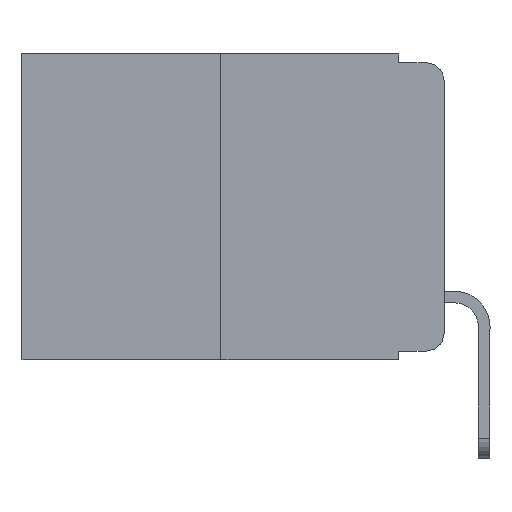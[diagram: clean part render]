
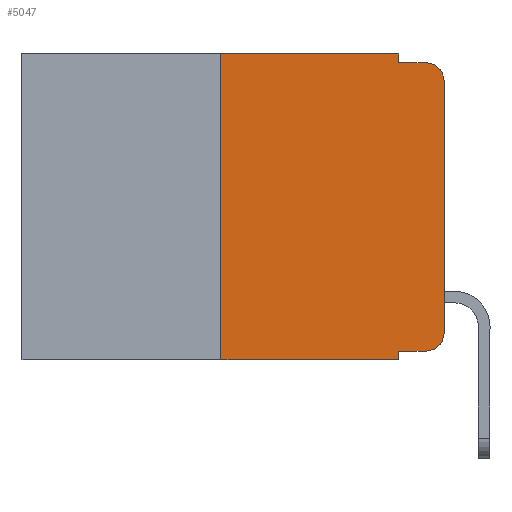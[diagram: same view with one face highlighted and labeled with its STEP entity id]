
A CAD part, left-side view. The second image highlights one B-rep face of the part: STEP entity #5047.
In plain terms, the highlighted planar face has unit normal (-1, 0, 0).
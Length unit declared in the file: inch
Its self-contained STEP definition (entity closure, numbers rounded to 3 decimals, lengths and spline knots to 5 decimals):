
#121 = VERTEX_POINT ( 'NONE', #5667 ) ;
#524 = LINE ( 'NONE', #859, #8742 ) ;
#543 = DIRECTION ( 'NONE',  ( -1., 0., 0. ) ) ;
#813 = DIRECTION ( 'NONE',  ( 0., 0., -1. ) ) ;
#859 = CARTESIAN_POINT ( 'NONE',  ( 0., 0.473, 0. ) ) ;
#891 = DIRECTION ( 'NONE',  ( 0., 0., -1. ) ) ;
#1900 = VERTEX_POINT ( 'NONE', #12485 ) ;
#2143 = LINE ( 'NONE', #16636, #10209 ) ;
#2450 = CARTESIAN_POINT ( 'NONE',  ( 0., 0.051, -0.01 ) ) ;
#2594 = ORIENTED_EDGE ( 'NONE', *, *, #8922, .F. ) ;
#2595 = DIRECTION ( 'NONE',  ( 1., 0., 0. ) ) ;
#3154 = VERTEX_POINT ( 'NONE', #13606 ) ;
#3578 = VERTEX_POINT ( 'NONE', #2450 ) ;
#3741 = LINE ( 'NONE', #18956, #18995 ) ;
#3841 = CARTESIAN_POINT ( 'NONE',  ( 0., 0.02, -0.01 ) ) ;
#3897 = AXIS2_PLACEMENT_3D ( 'NONE', #10343, #543, #11857 ) ;
#4141 = CARTESIAN_POINT ( 'NONE',  ( 0., 0.02, -0.03 ) ) ;
#4151 = ORIENTED_EDGE ( 'NONE', *, *, #8926, .F. ) ;
#5047 = ADVANCED_FACE ( 'NONE', ( #7954 ), #5959, .F. ) ;
#5652 = CARTESIAN_POINT ( 'NONE',  ( 0., 0.25, -0.343 ) ) ;
#5667 = CARTESIAN_POINT ( 'NONE',  ( 0., 0., -0.313 ) ) ;
#5697 = CARTESIAN_POINT ( 'NONE',  ( 0., 0., 0. ) ) ;
#5762 = DIRECTION ( 'NONE',  ( 0., 0., -1. ) ) ;
#5907 = CARTESIAN_POINT ( 'NONE',  ( 0., 0.051, -0.333 ) ) ;
#5959 = PLANE ( 'NONE',  #12268 ) ;
#6906 = ORIENTED_EDGE ( 'NONE', *, *, #8038, .F. ) ;
#7198 = VECTOR ( 'NONE', #7282, 39.37008 ) ;
#7282 = DIRECTION ( 'NONE',  ( 0., 0., 1. ) ) ;
#7420 = CARTESIAN_POINT ( 'NONE',  ( 0., 0.25, 0. ) ) ;
#7494 = VERTEX_POINT ( 'NONE', #10659 ) ;
#7954 = FACE_OUTER_BOUND ( 'NONE', #16239, .T. ) ;
#8038 = EDGE_CURVE ( 'NONE', #1900, #3154, #524, .T. ) ;
#8399 = ORIENTED_EDGE ( 'NONE', *, *, #8951, .T. ) ;
#8606 = LINE ( 'NONE', #7420, #13829 ) ;
#8622 = EDGE_CURVE ( 'NONE', #10189, #7494, #2143, .T. ) ;
#8742 = VECTOR ( 'NONE', #18988, 39.37008 ) ;
#8869 = EDGE_CURVE ( 'NONE', #121, #16444, #15114, .T. ) ;
#8894 = EDGE_CURVE ( 'NONE', #16444, #18422, #14265, .T. ) ;
#8897 = EDGE_CURVE ( 'NONE', #3578, #18422, #17869, .T. ) ;
#8922 = EDGE_CURVE ( 'NONE', #3154, #3578, #9420, .T. ) ;
#8925 = EDGE_CURVE ( 'NONE', #10189, #1900, #8606, .T. ) ;
#8926 = EDGE_CURVE ( 'NONE', #9802, #7494, #3741, .T. ) ;
#8951 = EDGE_CURVE ( 'NONE', #9802, #10324, #11674, .T. ) ;
#8952 = EDGE_CURVE ( 'NONE', #10324, #121, #14954, .T. ) ;
#9005 = DIRECTION ( 'NONE',  ( 0., 0., 1. ) ) ;
#9420 = LINE ( 'NONE', #13471, #17021 ) ;
#9636 = ORIENTED_EDGE ( 'NONE', *, *, #8869, .T. ) ;
#9802 = VERTEX_POINT ( 'NONE', #10296 ) ;
#10137 = ORIENTED_EDGE ( 'NONE', *, *, #8894, .T. ) ;
#10189 = VERTEX_POINT ( 'NONE', #5652 ) ;
#10209 = VECTOR ( 'NONE', #18006, 39.37008 ) ;
#10296 = CARTESIAN_POINT ( 'NONE',  ( 0., 0.051, -0.333 ) ) ;
#10324 = VERTEX_POINT ( 'NONE', #10920 ) ;
#10343 = CARTESIAN_POINT ( 'NONE',  ( 0., 0.02, -0.313 ) ) ;
#10659 = CARTESIAN_POINT ( 'NONE',  ( 0., 0.051, -0.343 ) ) ;
#10920 = CARTESIAN_POINT ( 'NONE',  ( 0., 0.02, -0.333 ) ) ;
#11218 = VECTOR ( 'NONE', #13531, 39.37008 ) ;
#11576 = ORIENTED_EDGE ( 'NONE', *, *, #8925, .F. ) ;
#11674 = LINE ( 'NONE', #5907, #11218 ) ;
#11857 = DIRECTION ( 'NONE',  ( 0., 0., -1. ) ) ;
#11992 = CARTESIAN_POINT ( 'NONE',  ( 0., 0.051, -0.01 ) ) ;
#12268 = AXIS2_PLACEMENT_3D ( 'NONE', #16314, #2595, #13513 ) ;
#12485 = CARTESIAN_POINT ( 'NONE',  ( 0., 0.25, 0. ) ) ;
#12922 = ORIENTED_EDGE ( 'NONE', *, *, #8952, .T. ) ;
#13471 = CARTESIAN_POINT ( 'NONE',  ( 0., 0.051, 0. ) ) ;
#13513 = DIRECTION ( 'NONE',  ( 0., 0., -1. ) ) ;
#13531 = DIRECTION ( 'NONE',  ( 0., -1., 0. ) ) ;
#13606 = CARTESIAN_POINT ( 'NONE',  ( 0., 0.051, 0. ) ) ;
#13829 = VECTOR ( 'NONE', #9005, 39.37008 ) ;
#14265 = CIRCLE ( 'NONE', #19103, 0.02 ) ;
#14799 = DIRECTION ( 'NONE',  ( -1., 0., 0. ) ) ;
#14954 = CIRCLE ( 'NONE', #3897, 0.02 ) ;
#15114 = LINE ( 'NONE', #5697, #7198 ) ;
#16239 = EDGE_LOOP ( 'NONE', ( #9636, #10137, #17622, #2594, #6906, #11576, #19345, #4151, #8399, #12922 ) ) ;
#16314 = CARTESIAN_POINT ( 'NONE',  ( 0., 0.473, 0. ) ) ;
#16444 = VERTEX_POINT ( 'NONE', #18553 ) ;
#16636 = CARTESIAN_POINT ( 'NONE',  ( 0., 0.473, -0.343 ) ) ;
#17021 = VECTOR ( 'NONE', #813, 39.37008 ) ;
#17438 = VECTOR ( 'NONE', #18831, 39.37008 ) ;
#17622 = ORIENTED_EDGE ( 'NONE', *, *, #8897, .F. ) ;
#17869 = LINE ( 'NONE', #11992, #17438 ) ;
#18006 = DIRECTION ( 'NONE',  ( 0., -1., 0. ) ) ;
#18422 = VERTEX_POINT ( 'NONE', #3841 ) ;
#18553 = CARTESIAN_POINT ( 'NONE',  ( 0., 0., -0.03 ) ) ;
#18831 = DIRECTION ( 'NONE',  ( 0., -1., 0. ) ) ;
#18956 = CARTESIAN_POINT ( 'NONE',  ( 0., 0.051, 0. ) ) ;
#18988 = DIRECTION ( 'NONE',  ( 0., -1., 0. ) ) ;
#18995 = VECTOR ( 'NONE', #891, 39.37008 ) ;
#19103 = AXIS2_PLACEMENT_3D ( 'NONE', #4141, #14799, #5762 ) ;
#19345 = ORIENTED_EDGE ( 'NONE', *, *, #8622, .T. ) ;
